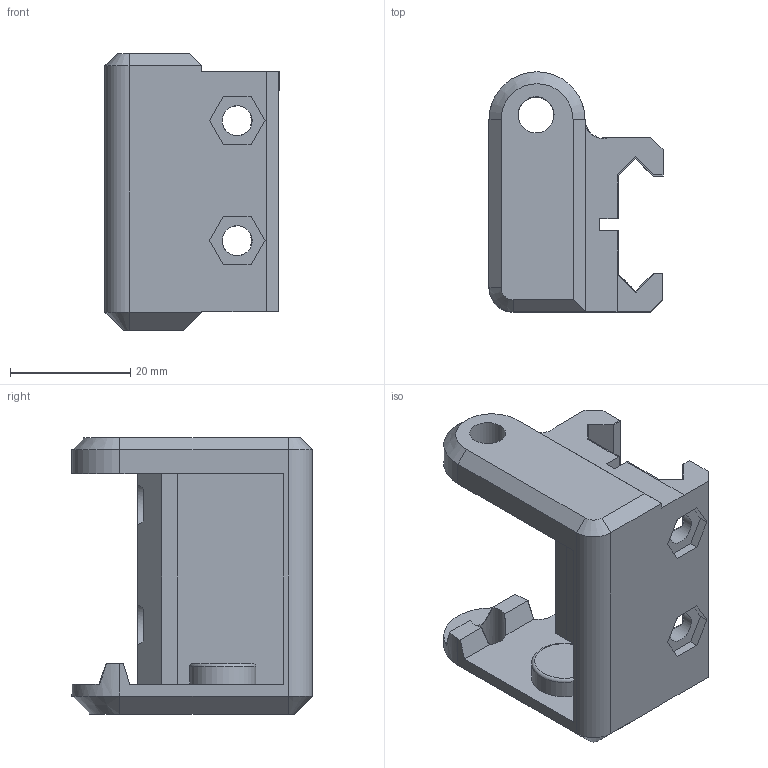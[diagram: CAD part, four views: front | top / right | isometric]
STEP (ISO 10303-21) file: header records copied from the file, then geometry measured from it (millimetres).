
FILE_DESCRIPTION(/* description */ (''),/* implementation_level */ '2;1');
FILE_NAME(/* name */ 'hinge.step',/* time_stamp */ '2021-09-02T19:32:09-05:00',/* author */ (''),/* organization */ (''),/* preprocessor_version */ 'ST-DEVELOPER v18.1',/* originating_system */ 'Autodesk Translation Framework v10.10.0.1391',/* authorisation */ '');
FILE_SCHEMA (('AUTOMOTIVE_DESIGN { 1 0 10303 214 3 1 1 }'));
Length unit declared in the file: millimetre
Products named in the file (1): new hinge
Bounding box: 28.99 x 40 x 46 mm (x, y, z)
Volume: 16805.6 mm3; surface area: 9143 mm2
Topology: 1 solids, 1 shells, 159 faces, 448 edges, 289 vertices
Faces by surface type: plane 121, bspline 21, cylinder 12, cone 4, torus 1
Full cylindrical faces by diameter (mm): 5 x4, 6 x2, 11 x1
Entity records: 5517 total; most frequent: CARTESIAN_POINT 1340, ORIENTED_EDGE 896, DIRECTION 840, EDGE_CURVE 448, LINE 310, VECTOR 310, VERTEX_POINT 289, AXIS2_PLACEMENT_3D 265
